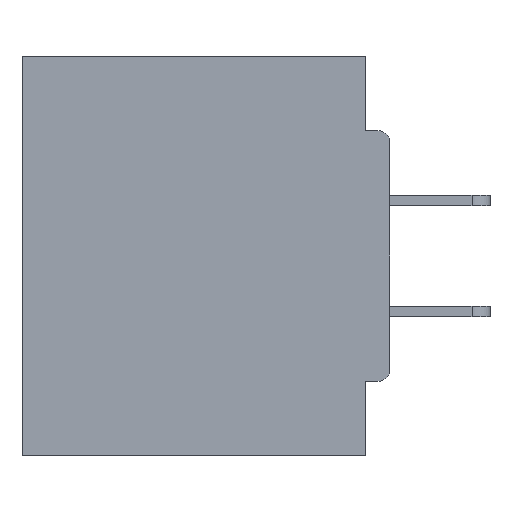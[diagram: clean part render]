
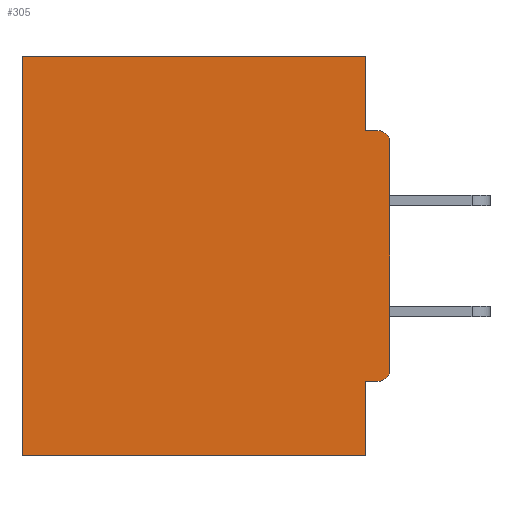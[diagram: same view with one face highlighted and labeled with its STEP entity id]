
A CAD part, left-side view. The second image highlights one B-rep face of the part: STEP entity #305.
In plain terms, the highlighted planar face has unit normal (-1, 0, 0).
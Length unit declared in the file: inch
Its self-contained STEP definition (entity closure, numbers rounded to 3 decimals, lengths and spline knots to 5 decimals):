
#39 = VERTEX_POINT ( 'NONE', #32896 ) ;
#151 = LINE ( 'NONE', #32232, #14573 ) ;
#305 = ADVANCED_FACE ( 'NONE', ( #2832 ), #11632, .F. ) ;
#453 = EDGE_CURVE ( 'NONE', #39, #23092, #151, .T. ) ;
#691 = CARTESIAN_POINT ( 'NONE',  ( 0.298, 0., -0.4065 ) ) ;
#2401 = LINE ( 'NONE', #28837, #35863 ) ;
#2832 = FACE_OUTER_BOUND ( 'NONE', #18657, .T. ) ;
#3563 = LINE ( 'NONE', #28950, #28813 ) ;
#4753 = AXIS2_PLACEMENT_3D ( 'NONE', #8765, #28941, #23007 ) ;
#5053 = VECTOR ( 'NONE', #8048, 39.37008 ) ;
#6135 = VECTOR ( 'NONE', #12131, 39.37008 ) ;
#6794 = DIRECTION ( 'NONE',  ( 0., 0., -1. ) ) ;
#6847 = VECTOR ( 'NONE', #6794, 39.37008 ) ;
#7354 = LINE ( 'NONE', #17404, #12299 ) ;
#7651 = CARTESIAN_POINT ( 'NONE',  ( 0.298, 0.031, -0.0935 ) ) ;
#8028 = EDGE_CURVE ( 'NONE', #33008, #36867, #34407, .T. ) ;
#8048 = DIRECTION ( 'NONE',  ( 0., 0., -1. ) ) ;
#8715 = DIRECTION ( 'NONE',  ( 0., 0., -1. ) ) ;
#8765 = CARTESIAN_POINT ( 'NONE',  ( 0.298, 0.015, -0.1085 ) ) ;
#9152 = VERTEX_POINT ( 'NONE', #33902 ) ;
#9304 = AXIS2_PLACEMENT_3D ( 'NONE', #30132, #24657, #12824 ) ;
#9940 = CARTESIAN_POINT ( 'NONE',  ( 0.298, 0.031, -0.5 ) ) ;
#10013 = CARTESIAN_POINT ( 'NONE',  ( 0.298, 0.46, 0. ) ) ;
#10268 = CARTESIAN_POINT ( 'NONE',  ( 0.298, 0.031, -0.5 ) ) ;
#10553 = ORIENTED_EDGE ( 'NONE', *, *, #12578, .T. ) ;
#11464 = ORIENTED_EDGE ( 'NONE', *, *, #453, .F. ) ;
#11632 = PLANE ( 'NONE',  #26900 ) ;
#11944 = DIRECTION ( 'NONE',  ( 0., -1., 0. ) ) ;
#12019 = DIRECTION ( 'NONE',  ( 0., 1., 0. ) ) ;
#12131 = DIRECTION ( 'NONE',  ( 0., 1., 0. ) ) ;
#12299 = VECTOR ( 'NONE', #8715, 39.37008 ) ;
#12578 = EDGE_CURVE ( 'NONE', #17368, #36263, #17167, .T. ) ;
#12824 = DIRECTION ( 'NONE',  ( 0., 0., -1. ) ) ;
#13227 = LINE ( 'NONE', #25429, #5053 ) ;
#13461 = EDGE_CURVE ( 'NONE', #39, #28689, #3563, .T. ) ;
#14361 = CARTESIAN_POINT ( 'NONE',  ( 0.298, 0.015, -0.0935 ) ) ;
#14412 = DIRECTION ( 'NONE',  ( 1., 0., 0. ) ) ;
#14573 = VECTOR ( 'NONE', #29691, 39.37008 ) ;
#15098 = EDGE_CURVE ( 'NONE', #36867, #9152, #24196, .T. ) ;
#16224 = ORIENTED_EDGE ( 'NONE', *, *, #22599, .F. ) ;
#16439 = EDGE_CURVE ( 'NONE', #23092, #36263, #2401, .T. ) ;
#17167 = CIRCLE ( 'NONE', #4753, 0.015 ) ;
#17225 = EDGE_CURVE ( 'NONE', #28689, #9152, #7354, .T. ) ;
#17368 = VERTEX_POINT ( 'NONE', #25893 ) ;
#17404 = CARTESIAN_POINT ( 'NONE',  ( 0.298, 0.46, 0. ) ) ;
#17553 = CARTESIAN_POINT ( 'NONE',  ( 0.298, 0., -0.5 ) ) ;
#17840 = DIRECTION ( 'NONE',  ( 0., 1., 0. ) ) ;
#18657 = EDGE_LOOP ( 'NONE', ( #10553, #24864, #11464, #23679, #20735, #29830, #27071, #21894, #31820, #16224 ) ) ;
#19321 = EDGE_CURVE ( 'NONE', #27606, #36699, #22892, .T. ) ;
#20348 = DIRECTION ( 'NONE',  ( 0., 0., -1. ) ) ;
#20735 = ORIENTED_EDGE ( 'NONE', *, *, #17225, .T. ) ;
#21894 = ORIENTED_EDGE ( 'NONE', *, *, #28527, .F. ) ;
#22599 = EDGE_CURVE ( 'NONE', #17368, #36699, #13227, .T. ) ;
#22892 = CIRCLE ( 'NONE', #9304, 0.015 ) ;
#23007 = DIRECTION ( 'NONE',  ( 0., 0., -1. ) ) ;
#23092 = VERTEX_POINT ( 'NONE', #7651 ) ;
#23679 = ORIENTED_EDGE ( 'NONE', *, *, #13461, .T. ) ;
#24196 = LINE ( 'NONE', #17553, #6135 ) ;
#24657 = DIRECTION ( 'NONE',  ( -1., 0., 0. ) ) ;
#24864 = ORIENTED_EDGE ( 'NONE', *, *, #16439, .F. ) ;
#25429 = CARTESIAN_POINT ( 'NONE',  ( 0.298, 0., 0. ) ) ;
#25893 = CARTESIAN_POINT ( 'NONE',  ( 0.298, 0., -0.1085 ) ) ;
#26537 = VECTOR ( 'NONE', #12019, 39.37008 ) ;
#26900 = AXIS2_PLACEMENT_3D ( 'NONE', #31719, #14412, #20348 ) ;
#27071 = ORIENTED_EDGE ( 'NONE', *, *, #8028, .F. ) ;
#27606 = VERTEX_POINT ( 'NONE', #28444 ) ;
#28444 = CARTESIAN_POINT ( 'NONE',  ( 0.298, 0.015, -0.4065 ) ) ;
#28527 = EDGE_CURVE ( 'NONE', #27606, #33008, #35183, .T. ) ;
#28689 = VERTEX_POINT ( 'NONE', #10013 ) ;
#28813 = VECTOR ( 'NONE', #17840, 39.37008 ) ;
#28837 = CARTESIAN_POINT ( 'NONE',  ( 0.298, 0., -0.0935 ) ) ;
#28941 = DIRECTION ( 'NONE',  ( -1., 0., 0. ) ) ;
#28950 = CARTESIAN_POINT ( 'NONE',  ( 0.298, 0., 0. ) ) ;
#29691 = DIRECTION ( 'NONE',  ( 0., 0., -1. ) ) ;
#29830 = ORIENTED_EDGE ( 'NONE', *, *, #15098, .F. ) ;
#30132 = CARTESIAN_POINT ( 'NONE',  ( 0.298, 0.015, -0.3915 ) ) ;
#31719 = CARTESIAN_POINT ( 'NONE',  ( 0.298, 0., 0. ) ) ;
#31820 = ORIENTED_EDGE ( 'NONE', *, *, #19321, .T. ) ;
#32232 = CARTESIAN_POINT ( 'NONE',  ( 0.298, 0.031, -0.5 ) ) ;
#32896 = CARTESIAN_POINT ( 'NONE',  ( 0.298, 0.031, 0. ) ) ;
#33008 = VERTEX_POINT ( 'NONE', #33440 ) ;
#33440 = CARTESIAN_POINT ( 'NONE',  ( 0.298, 0.031, -0.4065 ) ) ;
#33902 = CARTESIAN_POINT ( 'NONE',  ( 0.298, 0.46, -0.5 ) ) ;
#34407 = LINE ( 'NONE', #9940, #6847 ) ;
#35183 = LINE ( 'NONE', #691, #26537 ) ;
#35863 = VECTOR ( 'NONE', #11944, 39.37008 ) ;
#36263 = VERTEX_POINT ( 'NONE', #14361 ) ;
#36699 = VERTEX_POINT ( 'NONE', #37298 ) ;
#36867 = VERTEX_POINT ( 'NONE', #10268 ) ;
#37298 = CARTESIAN_POINT ( 'NONE',  ( 0.298, 0., -0.3915 ) ) ;
